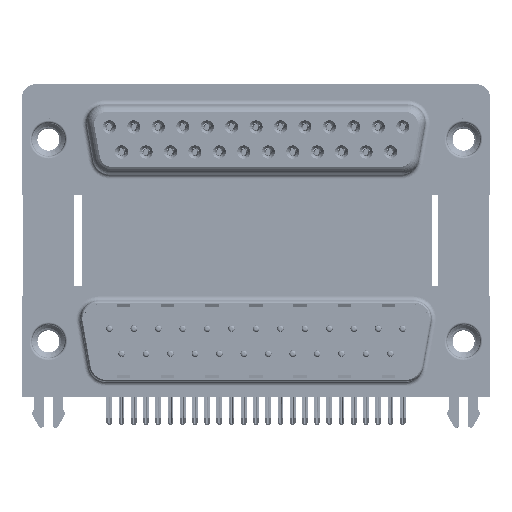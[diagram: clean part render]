
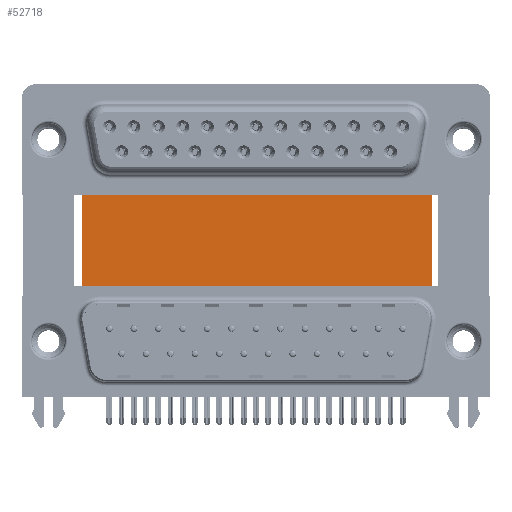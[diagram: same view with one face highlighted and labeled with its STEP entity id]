
A CAD part, top view. The second image highlights one B-rep face of the part: STEP entity #52718.
In plain terms, the highlighted planar face has unit normal (0, 0, 1).
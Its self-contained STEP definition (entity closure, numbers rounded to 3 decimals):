
#1603 = DIRECTION ( 'NONE',  ( 1., 0., 0. ) ) ;
#9077 = CARTESIAN_POINT ( 'NONE',  ( 43.43, -3.735, -12. ) ) ;
#12215 = VERTEX_POINT ( 'NONE', #25250 ) ;
#12620 = VECTOR ( 'NONE', #36462, 1000. ) ;
#14493 = CARTESIAN_POINT ( 'NONE',  ( 43.43, 16.585, -12. ) ) ;
#18253 = EDGE_CURVE ( 'NONE', #12215, #50307, #29568, .T. ) ;
#18957 = FACE_OUTER_BOUND ( 'NONE', #31284, .T. ) ;
#20100 = CARTESIAN_POINT ( 'NONE',  ( 3.79, 16.585, -12. ) ) ;
#23147 = DIRECTION ( 'NONE',  ( 0., -1., 0. ) ) ;
#24141 = CARTESIAN_POINT ( 'NONE',  ( 3.79, -3.735, -12. ) ) ;
#24391 = DIRECTION ( 'NONE',  ( 0., 0., -1. ) ) ;
#25250 = CARTESIAN_POINT ( 'NONE',  ( 3.79, -3.735, -12. ) ) ;
#25630 = VERTEX_POINT ( 'NONE', #34334 ) ;
#26373 = VECTOR ( 'NONE', #23147, 1000. ) ;
#29236 = ORIENTED_EDGE ( 'NONE', *, *, #37262, .F. ) ;
#29568 = LINE ( 'NONE', #24141, #35825 ) ;
#31193 = EDGE_CURVE ( 'NONE', #25630, #55564, #45903, .T. ) ;
#31284 = EDGE_LOOP ( 'NONE', ( #47356, #29236, #45177, #42849 ) ) ;
#32449 = PLANE ( 'NONE',  #54050 ) ;
#34334 = CARTESIAN_POINT ( 'NONE',  ( 3.79, 16.585, -12. ) ) ;
#35269 = EDGE_CURVE ( 'NONE', #25630, #12215, #45110, .T. ) ;
#35825 = VECTOR ( 'NONE', #50843, 1000. ) ;
#36462 = DIRECTION ( 'NONE',  ( 0., -1., 0. ) ) ;
#37262 = EDGE_CURVE ( 'NONE', #55564, #50307, #46135, .T. ) ;
#41950 = DIRECTION ( 'NONE',  ( -1., 0., 0. ) ) ;
#42149 = CARTESIAN_POINT ( 'NONE',  ( 3.79, 16.585, -12. ) ) ;
#42849 = ORIENTED_EDGE ( 'NONE', *, *, #35269, .T. ) ;
#45110 = LINE ( 'NONE', #53675, #12620 ) ;
#45177 = ORIENTED_EDGE ( 'NONE', *, *, #31193, .F. ) ;
#45903 = LINE ( 'NONE', #42149, #53142 ) ;
#46135 = LINE ( 'NONE', #14493, #26373 ) ;
#47356 = ORIENTED_EDGE ( 'NONE', *, *, #18253, .T. ) ;
#50307 = VERTEX_POINT ( 'NONE', #9077 ) ;
#50843 = DIRECTION ( 'NONE',  ( 1., 0., 0. ) ) ;
#52718 = ADVANCED_FACE ( 'NONE', ( #18957 ), #32449, .F. ) ;
#53142 = VECTOR ( 'NONE', #1603, 1000. ) ;
#53675 = CARTESIAN_POINT ( 'NONE',  ( 3.79, 16.585, -12. ) ) ;
#54050 = AXIS2_PLACEMENT_3D ( 'NONE', #20100, #24391, #41950 ) ;
#54759 = CARTESIAN_POINT ( 'NONE',  ( 43.43, 16.585, -12. ) ) ;
#55564 = VERTEX_POINT ( 'NONE', #54759 ) ;
